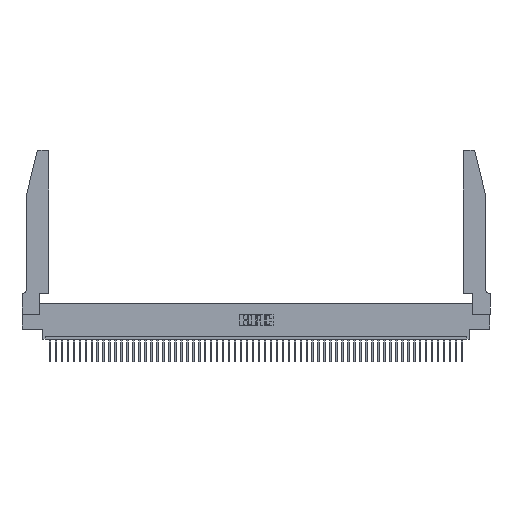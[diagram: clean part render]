
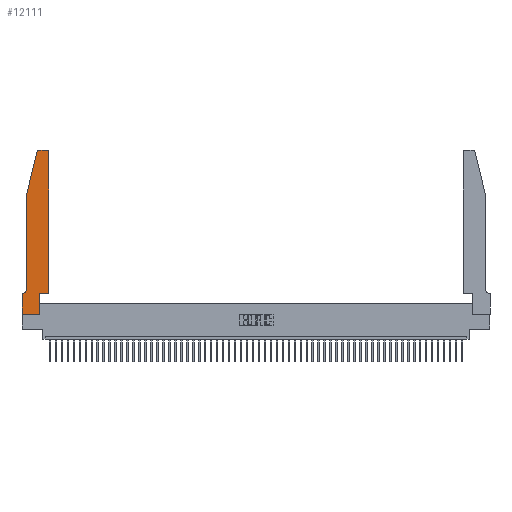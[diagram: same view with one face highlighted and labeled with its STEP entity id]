
A CAD part, top view. The second image highlights one B-rep face of the part: STEP entity #12111.
In plain terms, the highlighted planar face has unit normal (0, 0, 1).
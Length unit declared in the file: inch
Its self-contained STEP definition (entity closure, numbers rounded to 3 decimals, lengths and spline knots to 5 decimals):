
#515 = EDGE_CURVE ( 'NONE', #52950, #43281, #4574, .T. ) ;
#764 = CARTESIAN_POINT ( 'NONE',  ( 0.0055, 0.35, 0.37 ) ) ;
#805 = ORIENTED_EDGE ( 'NONE', *, *, #30660, .T. ) ;
#819 = VERTEX_POINT ( 'NONE', #24555 ) ;
#1255 = CARTESIAN_POINT ( 'NONE',  ( 0.284, 2.72, 0.37 ) ) ;
#1827 = DIRECTION ( 'NONE',  ( 1., 0., 0. ) ) ;
#3238 = EDGE_LOOP ( 'NONE', ( #16245, #42768, #38071, #47153, #51568, #805, #46415, #37180, #18635, #27278, #50690, #29346 ) ) ;
#3587 = VECTOR ( 'NONE', #18001, 39.37008 ) ;
#4574 = LINE ( 'NONE', #21399, #8519 ) ;
#4704 = DIRECTION ( 'NONE',  ( -1., 0., 0. ) ) ;
#4789 = EDGE_CURVE ( 'NONE', #53490, #24207, #29436, .T. ) ;
#4941 = CARTESIAN_POINT ( 'NONE',  ( 0.25487, 2.72718, 0.37 ) ) ;
#5609 = VERTEX_POINT ( 'NONE', #10960 ) ;
#6088 = CARTESIAN_POINT ( 'NONE',  ( 0.2865, 0., 0.37 ) ) ;
#6235 = CARTESIAN_POINT ( 'NONE',  ( 0.2865, 0.35, 0.37 ) ) ;
#6436 = CARTESIAN_POINT ( 'NONE',  ( 0.0055, 0.42, 0.37 ) ) ;
#6575 = AXIS2_PLACEMENT_3D ( 'NONE', #6436, #23129, #52190 ) ;
#8519 = VECTOR ( 'NONE', #4704, 39.37008 ) ;
#8612 = DIRECTION ( 'NONE',  ( 1., 0., 0. ) ) ;
#10281 = CARTESIAN_POINT ( 'NONE',  ( 0.4505, 0.35, 0.37 ) ) ;
#10366 = CARTESIAN_POINT ( 'NONE',  ( 0., 0., 0.37 ) ) ;
#10960 = CARTESIAN_POINT ( 'NONE',  ( 0.0755, 0.42, 0.37 ) ) ;
#11114 = AXIS2_PLACEMENT_3D ( 'NONE', #30227, #25578, #13757 ) ;
#12024 = CARTESIAN_POINT ( 'NONE',  ( 0., 0.35, 0.37 ) ) ;
#12029 = VECTOR ( 'NONE', #34611, 39.37008 ) ;
#12111 = ADVANCED_FACE ( 'NONE', ( #37749 ), #36882, .T. ) ;
#12421 = EDGE_CURVE ( 'NONE', #14236, #16599, #39089, .T. ) ;
#13009 = EDGE_CURVE ( 'NONE', #16599, #52950, #17013, .T. ) ;
#13016 = EDGE_CURVE ( 'NONE', #33888, #14236, #46200, .T. ) ;
#13757 = DIRECTION ( 'NONE',  ( 1., 0., 0. ) ) ;
#13816 = VECTOR ( 'NONE', #17561, 39.37008 ) ;
#14236 = VERTEX_POINT ( 'NONE', #25325 ) ;
#14343 = AXIS2_PLACEMENT_3D ( 'NONE', #1255, #39101, #1827 ) ;
#16205 = DIRECTION ( 'NONE',  ( 1., 0., 0. ) ) ;
#16245 = ORIENTED_EDGE ( 'NONE', *, *, #515, .T. ) ;
#16387 = VECTOR ( 'NONE', #30494, 39.37008 ) ;
#16541 = LINE ( 'NONE', #50771, #12029 ) ;
#16599 = VERTEX_POINT ( 'NONE', #49321 ) ;
#17013 = CIRCLE ( 'NONE', #11114, 0.03 ) ;
#17156 = LINE ( 'NONE', #42895, #3587 ) ;
#17561 = DIRECTION ( 'NONE',  ( 0., -1., 0. ) ) ;
#17720 = VECTOR ( 'NONE', #45234, 39.37008 ) ;
#18001 = DIRECTION ( 'NONE',  ( -1., 0., 0. ) ) ;
#18255 = EDGE_CURVE ( 'NONE', #43281, #45399, #53106, .T. ) ;
#18635 = ORIENTED_EDGE ( 'NONE', *, *, #35947, .T. ) ;
#19521 = CARTESIAN_POINT ( 'NONE',  ( 0.2865, 0.35, 0.37 ) ) ;
#20468 = VERTEX_POINT ( 'NONE', #764 ) ;
#21399 = CARTESIAN_POINT ( 'NONE',  ( 0.2605, 2.75, 0.37 ) ) ;
#21461 = AXIS2_PLACEMENT_3D ( 'NONE', #12024, #40327, #16205 ) ;
#22573 = EDGE_CURVE ( 'NONE', #45399, #819, #16541, .T. ) ;
#23129 = DIRECTION ( 'NONE',  ( 0., 0., -1. ) ) ;
#23460 = EDGE_CURVE ( 'NONE', #51864, #53490, #24934, .T. ) ;
#24207 = VERTEX_POINT ( 'NONE', #6088 ) ;
#24555 = CARTESIAN_POINT ( 'NONE',  ( 0.0755, 2., 0.37 ) ) ;
#24934 = LINE ( 'NONE', #34628, #13816 ) ;
#25325 = CARTESIAN_POINT ( 'NONE',  ( 0.4505, 0.35, 0.37 ) ) ;
#25478 = VECTOR ( 'NONE', #42844, 39.37008 ) ;
#25578 = DIRECTION ( 'NONE',  ( 0., 0., 1. ) ) ;
#27278 = ORIENTED_EDGE ( 'NONE', *, *, #13016, .T. ) ;
#29346 = ORIENTED_EDGE ( 'NONE', *, *, #13009, .T. ) ;
#29436 = LINE ( 'NONE', #37158, #43635 ) ;
#29805 = CARTESIAN_POINT ( 'NONE',  ( 0.4505, 0.35, 0.37 ) ) ;
#29984 = CARTESIAN_POINT ( 'NONE',  ( 0.284, 2.75, 0.37 ) ) ;
#30227 = CARTESIAN_POINT ( 'NONE',  ( 0.4205, 2.72, 0.37 ) ) ;
#30494 = DIRECTION ( 'NONE',  ( 0., -1., 0. ) ) ;
#30660 = EDGE_CURVE ( 'NONE', #20468, #51864, #17156, .T. ) ;
#30704 = LINE ( 'NONE', #19521, #17720 ) ;
#30978 = EDGE_CURVE ( 'NONE', #819, #5609, #43606, .T. ) ;
#33888 = VERTEX_POINT ( 'NONE', #6235 ) ;
#34611 = DIRECTION ( 'NONE',  ( -0.239, -0.971, 0. ) ) ;
#34628 = CARTESIAN_POINT ( 'NONE',  ( 0., 0., 0.37 ) ) ;
#34865 = CARTESIAN_POINT ( 'NONE',  ( 0.0755, 2., 0.37 ) ) ;
#35947 = EDGE_CURVE ( 'NONE', #24207, #33888, #30704, .T. ) ;
#36882 = PLANE ( 'NONE',  #21461 ) ;
#37158 = CARTESIAN_POINT ( 'NONE',  ( 0., 0., 0.37 ) ) ;
#37180 = ORIENTED_EDGE ( 'NONE', *, *, #4789, .T. ) ;
#37749 = FACE_OUTER_BOUND ( 'NONE', #3238, .T. ) ;
#38071 = ORIENTED_EDGE ( 'NONE', *, *, #22573, .T. ) ;
#39089 = LINE ( 'NONE', #29805, #25478 ) ;
#39101 = DIRECTION ( 'NONE',  ( 0., 0., 1. ) ) ;
#40327 = DIRECTION ( 'NONE',  ( 0., 0., 1. ) ) ;
#41121 = VECTOR ( 'NONE', #47098, 39.37008 ) ;
#41510 = EDGE_CURVE ( 'NONE', #5609, #20468, #51942, .T. ) ;
#42768 = ORIENTED_EDGE ( 'NONE', *, *, #18255, .T. ) ;
#42844 = DIRECTION ( 'NONE',  ( 0., 1., 0. ) ) ;
#42895 = CARTESIAN_POINT ( 'NONE',  ( 0.0755, 0.35, 0.37 ) ) ;
#43281 = VERTEX_POINT ( 'NONE', #29984 ) ;
#43606 = LINE ( 'NONE', #34865, #16387 ) ;
#43635 = VECTOR ( 'NONE', #8612, 39.37008 ) ;
#45234 = DIRECTION ( 'NONE',  ( 0., 1., 0. ) ) ;
#45399 = VERTEX_POINT ( 'NONE', #4941 ) ;
#45628 = CARTESIAN_POINT ( 'NONE',  ( 0., 0.35, 0.37 ) ) ;
#46200 = LINE ( 'NONE', #10281, #41121 ) ;
#46415 = ORIENTED_EDGE ( 'NONE', *, *, #23460, .T. ) ;
#47098 = DIRECTION ( 'NONE',  ( 1., 0., 0. ) ) ;
#47153 = ORIENTED_EDGE ( 'NONE', *, *, #30978, .T. ) ;
#47817 = CARTESIAN_POINT ( 'NONE',  ( 0.4205, 2.75, 0.37 ) ) ;
#49321 = CARTESIAN_POINT ( 'NONE',  ( 0.4505, 2.72, 0.37 ) ) ;
#50690 = ORIENTED_EDGE ( 'NONE', *, *, #12421, .T. ) ;
#50771 = CARTESIAN_POINT ( 'NONE',  ( 0.0755, 2., 0.37 ) ) ;
#51568 = ORIENTED_EDGE ( 'NONE', *, *, #41510, .T. ) ;
#51864 = VERTEX_POINT ( 'NONE', #45628 ) ;
#51942 = CIRCLE ( 'NONE', #6575, 0.07 ) ;
#52190 = DIRECTION ( 'NONE',  ( -1., 0., 0. ) ) ;
#52950 = VERTEX_POINT ( 'NONE', #47817 ) ;
#53106 = CIRCLE ( 'NONE', #14343, 0.03 ) ;
#53490 = VERTEX_POINT ( 'NONE', #10366 ) ;
